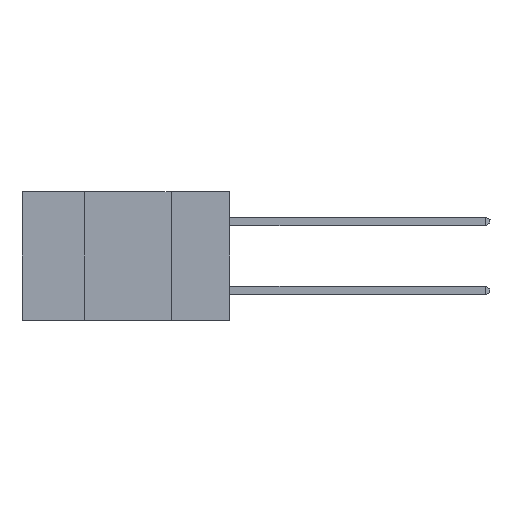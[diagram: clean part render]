
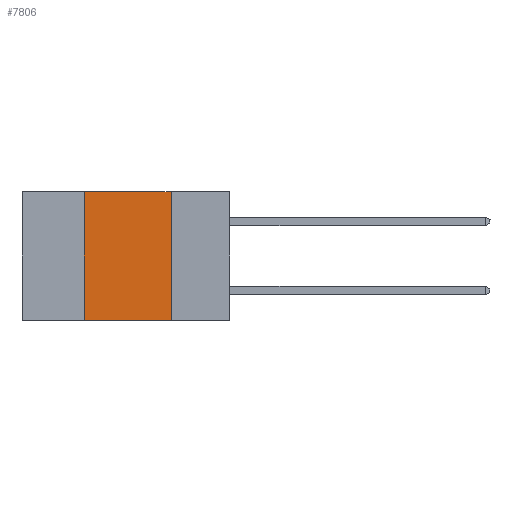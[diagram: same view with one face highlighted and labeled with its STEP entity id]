
A CAD part, left-side view. The second image highlights one B-rep face of the part: STEP entity #7806.
In plain terms, the highlighted planar face has unit normal (-1, 0, 0).
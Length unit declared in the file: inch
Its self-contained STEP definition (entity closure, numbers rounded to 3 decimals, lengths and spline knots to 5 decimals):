
#400 = FACE_OUTER_BOUND ( 'NONE', #4719, .T. ) ;
#2055 = LINE ( 'NONE', #9243, #11414 ) ;
#2475 = LINE ( 'NONE', #4165, #10286 ) ;
#2614 = AXIS2_PLACEMENT_3D ( 'NONE', #4081, #4445, #7930 ) ;
#2750 = DIRECTION ( 'NONE',  ( 0., -1., 0. ) ) ;
#2768 = EDGE_CURVE ( 'NONE', #10530, #6206, #2055, .T. ) ;
#2995 = LINE ( 'NONE', #8154, #8385 ) ;
#3327 = EDGE_CURVE ( 'NONE', #9091, #8519, #2475, .T. ) ;
#3603 = DIRECTION ( 'NONE',  ( 0., -1., 0. ) ) ;
#3730 = ORIENTED_EDGE ( 'NONE', *, *, #3327, .F. ) ;
#3819 = CARTESIAN_POINT ( 'NONE',  ( 0., 0.17, 0. ) ) ;
#4081 = CARTESIAN_POINT ( 'NONE',  ( 0., 0.6, 0. ) ) ;
#4165 = CARTESIAN_POINT ( 'NONE',  ( 0., 0.17, 0. ) ) ;
#4445 = DIRECTION ( 'NONE',  ( 1., 0., 0. ) ) ;
#4548 = EDGE_CURVE ( 'NONE', #6206, #9091, #7587, .T. ) ;
#4719 = EDGE_LOOP ( 'NONE', ( #3730, #6570, #6977, #11464 ) ) ;
#4831 = CARTESIAN_POINT ( 'NONE',  ( 0., 0.42, 0. ) ) ;
#4890 = VECTOR ( 'NONE', #3603, 39.37008 ) ;
#6010 = CARTESIAN_POINT ( 'NONE',  ( 0., 0.17, -0.37 ) ) ;
#6035 = DIRECTION ( 'NONE',  ( 0., 0., -1. ) ) ;
#6163 = CARTESIAN_POINT ( 'NONE',  ( 0., 0.42, -0.37 ) ) ;
#6206 = VERTEX_POINT ( 'NONE', #4831 ) ;
#6570 = ORIENTED_EDGE ( 'NONE', *, *, #4548, .F. ) ;
#6700 = EDGE_CURVE ( 'NONE', #10530, #8519, #2995, .T. ) ;
#6977 = ORIENTED_EDGE ( 'NONE', *, *, #2768, .F. ) ;
#7268 = CARTESIAN_POINT ( 'NONE',  ( 0., 0.6, 0. ) ) ;
#7587 = LINE ( 'NONE', #7268, #4890 ) ;
#7806 = ADVANCED_FACE ( 'NONE', ( #400 ), #9521, .F. ) ;
#7930 = DIRECTION ( 'NONE',  ( 0., 0., -1. ) ) ;
#8154 = CARTESIAN_POINT ( 'NONE',  ( 0., 0.6, -0.37 ) ) ;
#8385 = VECTOR ( 'NONE', #2750, 39.37008 ) ;
#8519 = VERTEX_POINT ( 'NONE', #6010 ) ;
#9091 = VERTEX_POINT ( 'NONE', #3819 ) ;
#9243 = CARTESIAN_POINT ( 'NONE',  ( 0., 0.42, 0. ) ) ;
#9521 = PLANE ( 'NONE',  #2614 ) ;
#10217 = DIRECTION ( 'NONE',  ( 0., 0., 1. ) ) ;
#10286 = VECTOR ( 'NONE', #6035, 39.37008 ) ;
#10530 = VERTEX_POINT ( 'NONE', #6163 ) ;
#11414 = VECTOR ( 'NONE', #10217, 39.37008 ) ;
#11464 = ORIENTED_EDGE ( 'NONE', *, *, #6700, .T. ) ;
